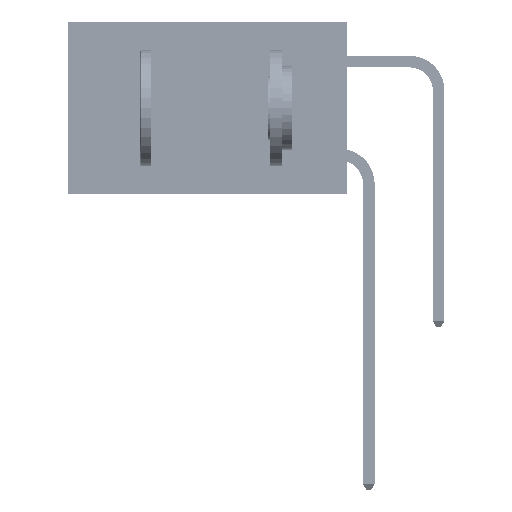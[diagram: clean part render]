
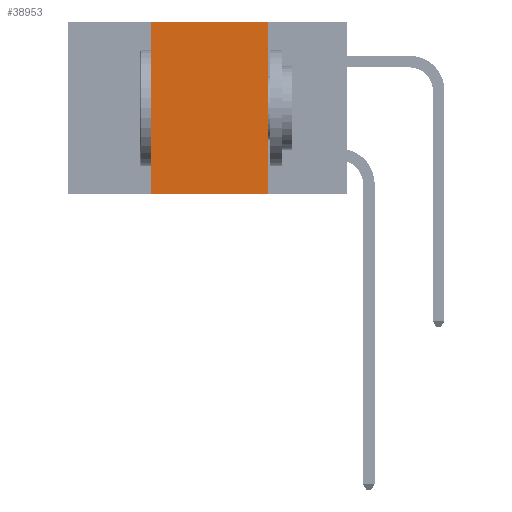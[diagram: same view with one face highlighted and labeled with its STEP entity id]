
A CAD part, left-side view. The second image highlights one B-rep face of the part: STEP entity #38953.
In plain terms, the highlighted planar face has unit normal (-1, 0, 0).
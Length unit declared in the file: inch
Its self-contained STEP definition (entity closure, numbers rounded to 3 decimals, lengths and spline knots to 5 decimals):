
#40 = CARTESIAN_POINT ( 'NONE',  ( 0., 0.42, 0. ) ) ;
#1607 = CARTESIAN_POINT ( 'NONE',  ( 0., 0.17, 0. ) ) ;
#2366 = CARTESIAN_POINT ( 'NONE',  ( 0., 0.17, 0. ) ) ;
#3703 = VERTEX_POINT ( 'NONE', #27780 ) ;
#4282 = VECTOR ( 'NONE', #12780, 39.37008 ) ;
#7135 = LINE ( 'NONE', #40, #17957 ) ;
#8431 = VERTEX_POINT ( 'NONE', #38449 ) ;
#9726 = DIRECTION ( 'NONE',  ( 1., 0., 0. ) ) ;
#9756 = LINE ( 'NONE', #2366, #29069 ) ;
#9986 = CARTESIAN_POINT ( 'NONE',  ( 0., 0.6, 0. ) ) ;
#12780 = DIRECTION ( 'NONE',  ( 0., -1., 0. ) ) ;
#14633 = ORIENTED_EDGE ( 'NONE', *, *, #16355, .F. ) ;
#15695 = VERTEX_POINT ( 'NONE', #17531 ) ;
#16355 = EDGE_CURVE ( 'NONE', #32091, #15695, #9756, .T. ) ;
#17531 = CARTESIAN_POINT ( 'NONE',  ( 0., 0.17, -0.37 ) ) ;
#17957 = VECTOR ( 'NONE', #25638, 39.37008 ) ;
#19767 = CARTESIAN_POINT ( 'NONE',  ( 0., 0.6, -0.37 ) ) ;
#20843 = CARTESIAN_POINT ( 'NONE',  ( 0., 0.6, 0. ) ) ;
#24164 = LINE ( 'NONE', #9986, #37818 ) ;
#25638 = DIRECTION ( 'NONE',  ( 0., 0., 1. ) ) ;
#27780 = CARTESIAN_POINT ( 'NONE',  ( 0., 0.42, -0.37 ) ) ;
#27799 = EDGE_LOOP ( 'NONE', ( #14633, #46790, #30840, #35890 ) ) ;
#29069 = VECTOR ( 'NONE', #46255, 39.37008 ) ;
#30052 = EDGE_CURVE ( 'NONE', #8431, #32091, #24164, .T. ) ;
#30840 = ORIENTED_EDGE ( 'NONE', *, *, #32944, .F. ) ;
#31341 = DIRECTION ( 'NONE',  ( 0., 0., -1. ) ) ;
#32091 = VERTEX_POINT ( 'NONE', #1607 ) ;
#32944 = EDGE_CURVE ( 'NONE', #3703, #8431, #7135, .T. ) ;
#33417 = AXIS2_PLACEMENT_3D ( 'NONE', #20843, #9726, #31341 ) ;
#34994 = LINE ( 'NONE', #19767, #4282 ) ;
#35890 = ORIENTED_EDGE ( 'NONE', *, *, #42306, .T. ) ;
#37818 = VECTOR ( 'NONE', #39067, 39.37008 ) ;
#38449 = CARTESIAN_POINT ( 'NONE',  ( 0., 0.42, 0. ) ) ;
#38953 = ADVANCED_FACE ( 'NONE', ( #40415 ), #46438, .F. ) ;
#39067 = DIRECTION ( 'NONE',  ( 0., -1., 0. ) ) ;
#40415 = FACE_OUTER_BOUND ( 'NONE', #27799, .T. ) ;
#42306 = EDGE_CURVE ( 'NONE', #3703, #15695, #34994, .T. ) ;
#46255 = DIRECTION ( 'NONE',  ( 0., 0., -1. ) ) ;
#46438 = PLANE ( 'NONE',  #33417 ) ;
#46790 = ORIENTED_EDGE ( 'NONE', *, *, #30052, .F. ) ;
